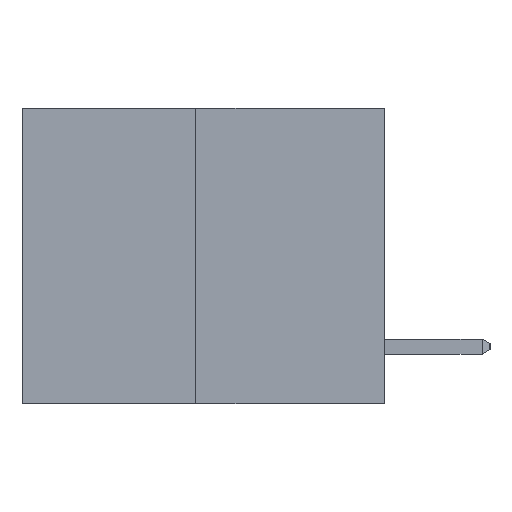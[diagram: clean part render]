
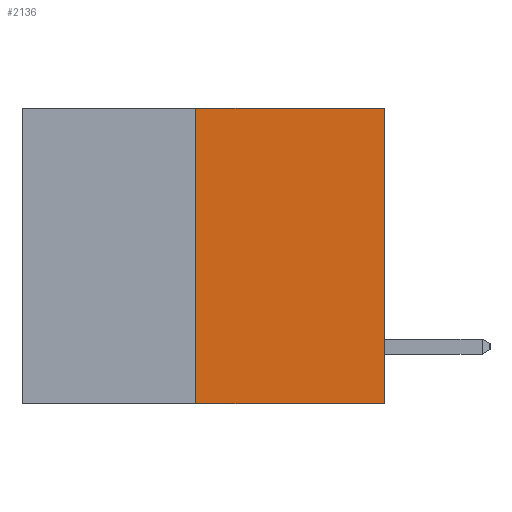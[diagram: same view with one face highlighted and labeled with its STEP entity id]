
A CAD part, left-side view. The second image highlights one B-rep face of the part: STEP entity #2136.
In plain terms, the highlighted planar face has unit normal (-1, 0, 0).
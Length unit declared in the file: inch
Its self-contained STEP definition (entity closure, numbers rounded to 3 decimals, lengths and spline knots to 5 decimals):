
#106 = LINE ( 'NONE', #3408, #8685 ) ;
#207 = EDGE_CURVE ( 'NONE', #5633, #8741, #106, .T. ) ;
#575 = CARTESIAN_POINT ( 'NONE',  ( 0., 0.6, -0.49 ) ) ;
#710 = DIRECTION ( 'NONE',  ( 0., -1., 0. ) ) ;
#801 = ORIENTED_EDGE ( 'NONE', *, *, #207, .F. ) ;
#967 = VERTEX_POINT ( 'NONE', #12345 ) ;
#2136 = ADVANCED_FACE ( 'NONE', ( #11442 ), #9757, .F. ) ;
#2919 = CARTESIAN_POINT ( 'NONE',  ( 0., 0.6, 0. ) ) ;
#3408 = CARTESIAN_POINT ( 'NONE',  ( 0., 0.312, -0.49 ) ) ;
#3917 = DIRECTION ( 'NONE',  ( 0., -1., 0. ) ) ;
#4149 = AXIS2_PLACEMENT_3D ( 'NONE', #4729, #7702, #11771 ) ;
#4366 = CARTESIAN_POINT ( 'NONE',  ( 0., 0., -0.49 ) ) ;
#4540 = EDGE_CURVE ( 'NONE', #5633, #8406, #5488, .T. ) ;
#4701 = VECTOR ( 'NONE', #710, 39.37008 ) ;
#4729 = CARTESIAN_POINT ( 'NONE',  ( 0., 0.6, 0. ) ) ;
#4972 = DIRECTION ( 'NONE',  ( 0., 0., 1. ) ) ;
#5089 = CARTESIAN_POINT ( 'NONE',  ( 0., 0.312, 0. ) ) ;
#5488 = LINE ( 'NONE', #575, #4701 ) ;
#5545 = VECTOR ( 'NONE', #4972, 39.37008 ) ;
#5633 = VERTEX_POINT ( 'NONE', #11203 ) ;
#5847 = CARTESIAN_POINT ( 'NONE',  ( 0., 0., 0. ) ) ;
#6312 = ORIENTED_EDGE ( 'NONE', *, *, #8680, .T. ) ;
#6985 = VECTOR ( 'NONE', #3917, 39.37008 ) ;
#7099 = ORIENTED_EDGE ( 'NONE', *, *, #7370, .F. ) ;
#7370 = EDGE_CURVE ( 'NONE', #8741, #967, #10876, .T. ) ;
#7702 = DIRECTION ( 'NONE',  ( 1., 0., 0. ) ) ;
#8203 = LINE ( 'NONE', #5847, #5545 ) ;
#8338 = DIRECTION ( 'NONE',  ( 0., 0., 1. ) ) ;
#8406 = VERTEX_POINT ( 'NONE', #4366 ) ;
#8680 = EDGE_CURVE ( 'NONE', #8406, #967, #8203, .T. ) ;
#8685 = VECTOR ( 'NONE', #8338, 39.37008 ) ;
#8741 = VERTEX_POINT ( 'NONE', #5089 ) ;
#9445 = EDGE_LOOP ( 'NONE', ( #801, #9619, #6312, #7099 ) ) ;
#9619 = ORIENTED_EDGE ( 'NONE', *, *, #4540, .T. ) ;
#9757 = PLANE ( 'NONE',  #4149 ) ;
#10876 = LINE ( 'NONE', #2919, #6985 ) ;
#11203 = CARTESIAN_POINT ( 'NONE',  ( 0., 0.312, -0.49 ) ) ;
#11442 = FACE_OUTER_BOUND ( 'NONE', #9445, .T. ) ;
#11771 = DIRECTION ( 'NONE',  ( 0., 0., -1. ) ) ;
#12345 = CARTESIAN_POINT ( 'NONE',  ( 0., 0., 0. ) ) ;
